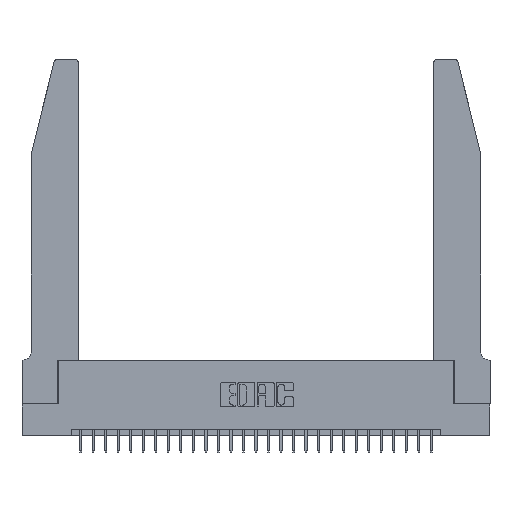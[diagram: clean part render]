
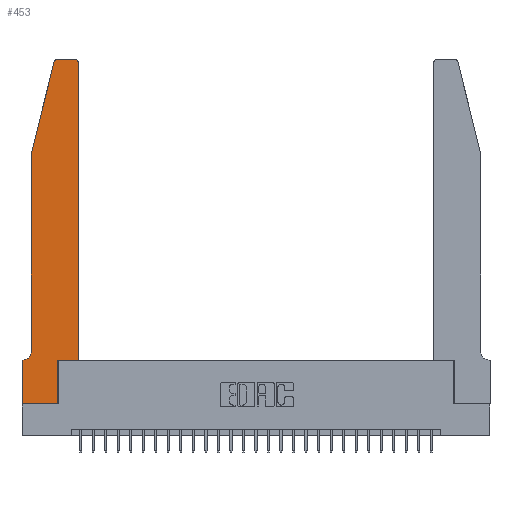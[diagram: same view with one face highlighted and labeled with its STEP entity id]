
A CAD part, top view. The second image highlights one B-rep face of the part: STEP entity #453.
In plain terms, the highlighted planar face has unit normal (0, 0, 1).
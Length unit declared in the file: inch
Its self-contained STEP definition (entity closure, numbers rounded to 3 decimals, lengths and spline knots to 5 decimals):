
#453 = ADVANCED_FACE ( 'NONE', ( #29144 ), #15574, .T. ) ;
#523 = LINE ( 'NONE', #27978, #2211 ) ;
#942 = LINE ( 'NONE', #14241, #13112 ) ;
#1070 = VERTEX_POINT ( 'NONE', #22793 ) ;
#1232 = CARTESIAN_POINT ( 'NONE',  ( 0.284, 2.75, 0.37 ) ) ;
#1751 = ORIENTED_EDGE ( 'NONE', *, *, #8716, .T. ) ;
#2011 = VECTOR ( 'NONE', #22006, 39.37008 ) ;
#2207 = DIRECTION ( 'NONE',  ( 1., 0., 0. ) ) ;
#2211 = VECTOR ( 'NONE', #23660, 39.37008 ) ;
#2634 = CARTESIAN_POINT ( 'NONE',  ( 0.4205, 2.72, 0.37 ) ) ;
#2735 = LINE ( 'NONE', #11764, #19911 ) ;
#3950 = CARTESIAN_POINT ( 'NONE',  ( 0.2865, 0.35, 0.37 ) ) ;
#4194 = CIRCLE ( 'NONE', #15541, 0.03 ) ;
#4421 = LINE ( 'NONE', #22530, #7963 ) ;
#4934 = CARTESIAN_POINT ( 'NONE',  ( 0.0055, 0.42, 0.37 ) ) ;
#5317 = DIRECTION ( 'NONE',  ( 1., 0., 0. ) ) ;
#5420 = ORIENTED_EDGE ( 'NONE', *, *, #27610, .T. ) ;
#5460 = AXIS2_PLACEMENT_3D ( 'NONE', #27188, #24645, #11430 ) ;
#5757 = CARTESIAN_POINT ( 'NONE',  ( 0.4505, 0.35, 0.37 ) ) ;
#6013 = LINE ( 'NONE', #9846, #12956 ) ;
#7013 = VECTOR ( 'NONE', #13441, 39.37008 ) ;
#7683 = ORIENTED_EDGE ( 'NONE', *, *, #17965, .T. ) ;
#7963 = VECTOR ( 'NONE', #2207, 39.37008 ) ;
#8123 = VERTEX_POINT ( 'NONE', #8993 ) ;
#8704 = LINE ( 'NONE', #13137, #19501 ) ;
#8716 = EDGE_CURVE ( 'NONE', #9165, #14766, #21362, .T. ) ;
#8726 = CARTESIAN_POINT ( 'NONE',  ( 0.0055, 0.35, 0.37 ) ) ;
#8993 = CARTESIAN_POINT ( 'NONE',  ( 0.4505, 2.72, 0.37 ) ) ;
#9165 = VERTEX_POINT ( 'NONE', #19091 ) ;
#9310 = EDGE_CURVE ( 'NONE', #1070, #18390, #8704, .T. ) ;
#9846 = CARTESIAN_POINT ( 'NONE',  ( 0., 0., 0.37 ) ) ;
#10237 = CARTESIAN_POINT ( 'NONE',  ( 0.2865, 0., 0.37 ) ) ;
#10651 = VERTEX_POINT ( 'NONE', #3950 ) ;
#10869 = AXIS2_PLACEMENT_3D ( 'NONE', #4934, #13953, #23031 ) ;
#10950 = CARTESIAN_POINT ( 'NONE',  ( 0.4505, 0.35, 0.37 ) ) ;
#11117 = EDGE_CURVE ( 'NONE', #25463, #11246, #24094, .T. ) ;
#11161 = CARTESIAN_POINT ( 'NONE',  ( 0.0755, 0.42, 0.37 ) ) ;
#11246 = VERTEX_POINT ( 'NONE', #11161 ) ;
#11430 = DIRECTION ( 'NONE',  ( 1., 0., 0. ) ) ;
#11764 = CARTESIAN_POINT ( 'NONE',  ( 0.0755, 2., 0.37 ) ) ;
#11961 = DIRECTION ( 'NONE',  ( 0., 0., 1. ) ) ;
#12014 = VERTEX_POINT ( 'NONE', #25310 ) ;
#12794 = CARTESIAN_POINT ( 'NONE',  ( 0.0755, 2., 0.37 ) ) ;
#12956 = VECTOR ( 'NONE', #19638, 39.37008 ) ;
#13112 = VECTOR ( 'NONE', #21246, 39.37008 ) ;
#13137 = CARTESIAN_POINT ( 'NONE',  ( 0.2605, 2.75, 0.37 ) ) ;
#13441 = DIRECTION ( 'NONE',  ( 0., 1., 0. ) ) ;
#13907 = CIRCLE ( 'NONE', #21527, 0.03 ) ;
#13953 = DIRECTION ( 'NONE',  ( 0., 0., -1. ) ) ;
#14241 = CARTESIAN_POINT ( 'NONE',  ( 0.0755, 0.35, 0.37 ) ) ;
#14766 = VERTEX_POINT ( 'NONE', #10237 ) ;
#15355 = VERTEX_POINT ( 'NONE', #23749 ) ;
#15541 = AXIS2_PLACEMENT_3D ( 'NONE', #2634, #11961, #5317 ) ;
#15574 = PLANE ( 'NONE',  #5460 ) ;
#15934 = EDGE_CURVE ( 'NONE', #24096, #15355, #942, .T. ) ;
#16635 = EDGE_CURVE ( 'NONE', #14766, #10651, #523, .T. ) ;
#16760 = CARTESIAN_POINT ( 'NONE',  ( 0., 0., 0.37 ) ) ;
#16865 = ORIENTED_EDGE ( 'NONE', *, *, #19022, .T. ) ;
#17311 = DIRECTION ( 'NONE',  ( -1., 0., 0. ) ) ;
#17845 = EDGE_CURVE ( 'NONE', #24380, #8123, #24604, .T. ) ;
#17965 = EDGE_CURVE ( 'NONE', #10651, #24380, #4421, .T. ) ;
#18154 = ORIENTED_EDGE ( 'NONE', *, *, #16635, .T. ) ;
#18390 = VERTEX_POINT ( 'NONE', #1232 ) ;
#19022 = EDGE_CURVE ( 'NONE', #8123, #1070, #4194, .T. ) ;
#19091 = CARTESIAN_POINT ( 'NONE',  ( 0., 0., 0.37 ) ) ;
#19126 = DIRECTION ( 'NONE',  ( 1., 0., 0. ) ) ;
#19501 = VECTOR ( 'NONE', #17311, 39.37008 ) ;
#19638 = DIRECTION ( 'NONE',  ( 0., -1., 0. ) ) ;
#19679 = ORIENTED_EDGE ( 'NONE', *, *, #19924, .T. ) ;
#19911 = VECTOR ( 'NONE', #20823, 39.37008 ) ;
#19924 = EDGE_CURVE ( 'NONE', #11246, #24096, #25076, .T. ) ;
#20393 = ORIENTED_EDGE ( 'NONE', *, *, #23043, .T. ) ;
#20823 = DIRECTION ( 'NONE',  ( -0.239, -0.971, 0. ) ) ;
#21060 = DIRECTION ( 'NONE',  ( 1., 0., 0. ) ) ;
#21246 = DIRECTION ( 'NONE',  ( -1., 0., 0. ) ) ;
#21362 = LINE ( 'NONE', #16760, #27919 ) ;
#21527 = AXIS2_PLACEMENT_3D ( 'NONE', #21665, #28381, #21060 ) ;
#21657 = ORIENTED_EDGE ( 'NONE', *, *, #17845, .T. ) ;
#21665 = CARTESIAN_POINT ( 'NONE',  ( 0.284, 2.72, 0.37 ) ) ;
#21764 = ORIENTED_EDGE ( 'NONE', *, *, #28284, .T. ) ;
#22006 = DIRECTION ( 'NONE',  ( 0., -1., 0. ) ) ;
#22530 = CARTESIAN_POINT ( 'NONE',  ( 0.4505, 0.35, 0.37 ) ) ;
#22793 = CARTESIAN_POINT ( 'NONE',  ( 0.4205, 2.75, 0.37 ) ) ;
#23031 = DIRECTION ( 'NONE',  ( -1., 0., 0. ) ) ;
#23043 = EDGE_CURVE ( 'NONE', #12014, #25463, #2735, .T. ) ;
#23660 = DIRECTION ( 'NONE',  ( 0., 1., 0. ) ) ;
#23749 = CARTESIAN_POINT ( 'NONE',  ( 0., 0.35, 0.37 ) ) ;
#24094 = LINE ( 'NONE', #12794, #2011 ) ;
#24096 = VERTEX_POINT ( 'NONE', #8726 ) ;
#24380 = VERTEX_POINT ( 'NONE', #5757 ) ;
#24604 = LINE ( 'NONE', #10950, #7013 ) ;
#24645 = DIRECTION ( 'NONE',  ( 0., 0., 1. ) ) ;
#24982 = EDGE_LOOP ( 'NONE', ( #28447, #21764, #20393, #27634, #19679, #26676, #5420, #1751, #18154, #7683, #21657, #16865 ) ) ;
#25071 = CARTESIAN_POINT ( 'NONE',  ( 0.0755, 2., 0.37 ) ) ;
#25076 = CIRCLE ( 'NONE', #10869, 0.07 ) ;
#25310 = CARTESIAN_POINT ( 'NONE',  ( 0.25487, 2.72718, 0.37 ) ) ;
#25463 = VERTEX_POINT ( 'NONE', #25071 ) ;
#26676 = ORIENTED_EDGE ( 'NONE', *, *, #15934, .T. ) ;
#27188 = CARTESIAN_POINT ( 'NONE',  ( 0., 0.35, 0.37 ) ) ;
#27610 = EDGE_CURVE ( 'NONE', #15355, #9165, #6013, .T. ) ;
#27634 = ORIENTED_EDGE ( 'NONE', *, *, #11117, .T. ) ;
#27919 = VECTOR ( 'NONE', #19126, 39.37008 ) ;
#27978 = CARTESIAN_POINT ( 'NONE',  ( 0.2865, 0.35, 0.37 ) ) ;
#28284 = EDGE_CURVE ( 'NONE', #18390, #12014, #13907, .T. ) ;
#28381 = DIRECTION ( 'NONE',  ( 0., 0., 1. ) ) ;
#28447 = ORIENTED_EDGE ( 'NONE', *, *, #9310, .T. ) ;
#29144 = FACE_OUTER_BOUND ( 'NONE', #24982, .T. ) ;
